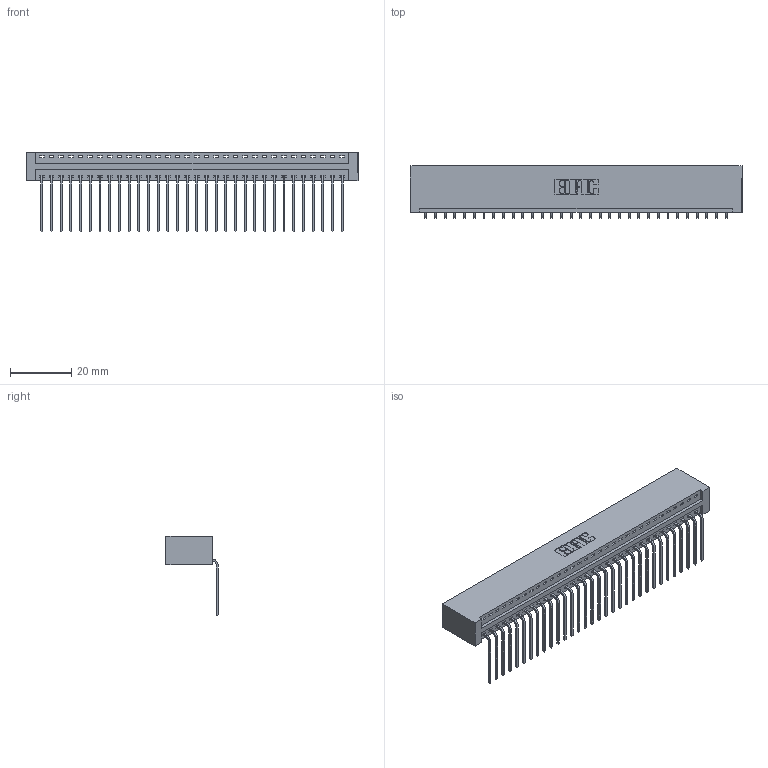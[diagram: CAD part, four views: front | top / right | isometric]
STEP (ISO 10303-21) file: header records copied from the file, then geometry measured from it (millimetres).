
FILE_DESCRIPTION (( 'STEP AP203' ), '1' );
FILE_NAME ('346-032-559-101.STEP', '2018-08-22T10:08:23', ( '' ), ( '' ), 'SwSTEP 2.0', 'SolidWorks 2016', '' );
FILE_SCHEMA (( 'CONFIG_CONTROL_DESIGN' ));
Length unit declared in the file: inch
Products named in the file (3): 346 Part_No Mounting Lugs; 345-292-001_558 559 Tail - 1; 346-032-559-101
Assembly tree (33 placements, depth 2):
  346-032-559-101
    346 Part_No Mounting Lugs
    345-292-001_558 559 Tail - 1  x32
Bounding box: 108.84 x 17.08 x 26.16 mm (x, y, z)
Volume: 11005.4 mm3; surface area: 14358.6 mm2
Topology: 33 solids, 33 shells, 2034 faces, 6129 edges, 4042 vertices
Faces by surface type: plane 1416, cylinder 618
Entity records: 21013 total; most frequent: CARTESIAN_POINT 3612, ORIENTED_EDGE 3578, DIRECTION 3193, EDGE_CURVE 1789, LINE 1537, VECTOR 1537, VERTEX_POINT 1190, AXIS2_PLACEMENT_3D 828
